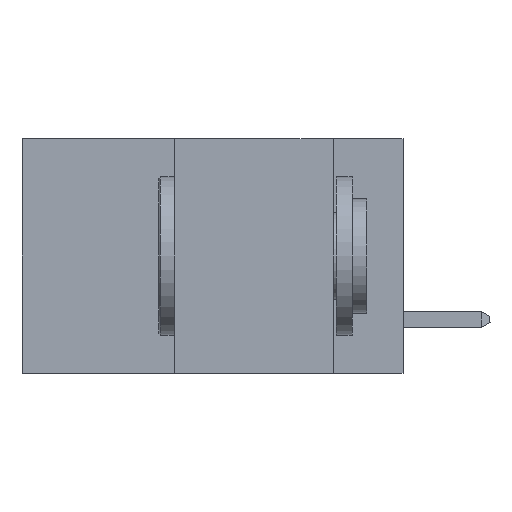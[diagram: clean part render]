
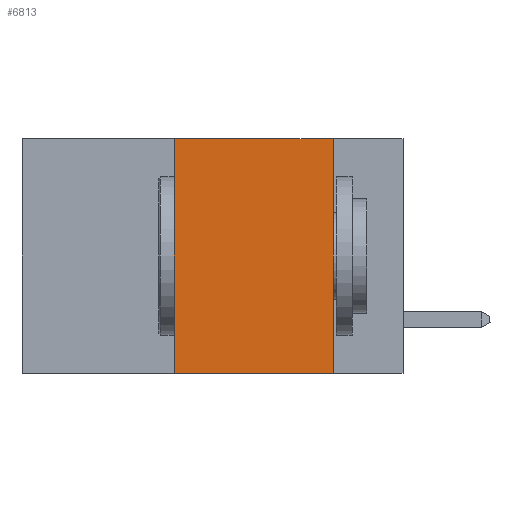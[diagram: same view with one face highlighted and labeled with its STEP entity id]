
A CAD part, left-side view. The second image highlights one B-rep face of the part: STEP entity #6813.
In plain terms, the highlighted planar face has unit normal (-1, 0, 0).
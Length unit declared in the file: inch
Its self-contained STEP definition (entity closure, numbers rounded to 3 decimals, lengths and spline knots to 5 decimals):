
#1360 = VERTEX_POINT ( 'NONE', #7317 ) ;
#3193 = VERTEX_POINT ( 'NONE', #29683 ) ;
#4294 = DIRECTION ( 'NONE',  ( 0., 0., 1. ) ) ;
#4784 = VERTEX_POINT ( 'NONE', #19074 ) ;
#5551 = ORIENTED_EDGE ( 'NONE', *, *, #32063, .F. ) ;
#5704 = VECTOR ( 'NONE', #20062, 39.37008 ) ;
#6813 = ADVANCED_FACE ( 'NONE', ( #8963 ), #22461, .F. ) ;
#7317 = CARTESIAN_POINT ( 'NONE',  ( 0., 0.36, 0. ) ) ;
#8963 = FACE_OUTER_BOUND ( 'NONE', #28093, .T. ) ;
#9045 = DIRECTION ( 'NONE',  ( 0., 0., -1. ) ) ;
#13722 = ORIENTED_EDGE ( 'NONE', *, *, #26597, .F. ) ;
#13773 = DIRECTION ( 'NONE',  ( 0., -1., 0. ) ) ;
#15671 = VECTOR ( 'NONE', #13773, 39.37008 ) ;
#16442 = CARTESIAN_POINT ( 'NONE',  ( 0., 0.11, -0.37 ) ) ;
#17101 = CARTESIAN_POINT ( 'NONE',  ( 0., 0.6, 0. ) ) ;
#17126 = CARTESIAN_POINT ( 'NONE',  ( 0., 0.6, -0.37 ) ) ;
#17386 = CARTESIAN_POINT ( 'NONE',  ( 0., 0.11, 0. ) ) ;
#17945 = ORIENTED_EDGE ( 'NONE', *, *, #34259, .F. ) ;
#19074 = CARTESIAN_POINT ( 'NONE',  ( 0., 0.11, 0. ) ) ;
#19800 = DIRECTION ( 'NONE',  ( 0., -1., 0. ) ) ;
#20062 = DIRECTION ( 'NONE',  ( 0., 0., -1. ) ) ;
#20523 = CARTESIAN_POINT ( 'NONE',  ( 0., 0.36, 0. ) ) ;
#20705 = VECTOR ( 'NONE', #19800, 39.37008 ) ;
#22461 = PLANE ( 'NONE',  #24226 ) ;
#24226 = AXIS2_PLACEMENT_3D ( 'NONE', #17101, #25157, #9045 ) ;
#25157 = DIRECTION ( 'NONE',  ( 1., 0., 0. ) ) ;
#26597 = EDGE_CURVE ( 'NONE', #3193, #1360, #34038, .T. ) ;
#27016 = LINE ( 'NONE', #17126, #20705 ) ;
#27069 = EDGE_CURVE ( 'NONE', #3193, #33297, #27016, .T. ) ;
#27346 = ORIENTED_EDGE ( 'NONE', *, *, #27069, .T. ) ;
#27902 = VECTOR ( 'NONE', #4294, 39.37008 ) ;
#28088 = LINE ( 'NONE', #17386, #5704 ) ;
#28093 = EDGE_LOOP ( 'NONE', ( #17945, #5551, #13722, #27346 ) ) ;
#29083 = LINE ( 'NONE', #29853, #15671 ) ;
#29683 = CARTESIAN_POINT ( 'NONE',  ( 0., 0.36, -0.37 ) ) ;
#29853 = CARTESIAN_POINT ( 'NONE',  ( 0., 0.6, 0. ) ) ;
#32063 = EDGE_CURVE ( 'NONE', #1360, #4784, #29083, .T. ) ;
#33297 = VERTEX_POINT ( 'NONE', #16442 ) ;
#34038 = LINE ( 'NONE', #20523, #27902 ) ;
#34259 = EDGE_CURVE ( 'NONE', #4784, #33297, #28088, .T. ) ;
